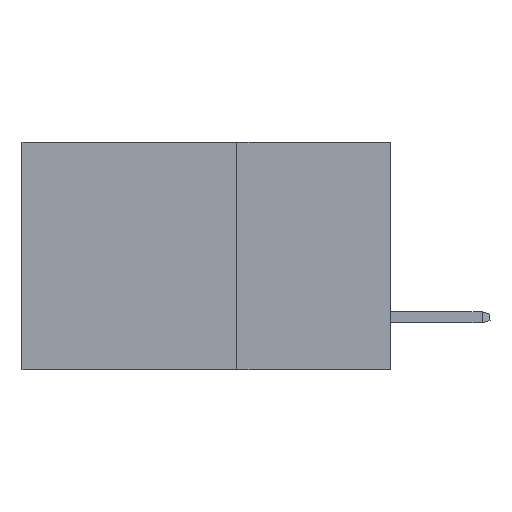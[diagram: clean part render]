
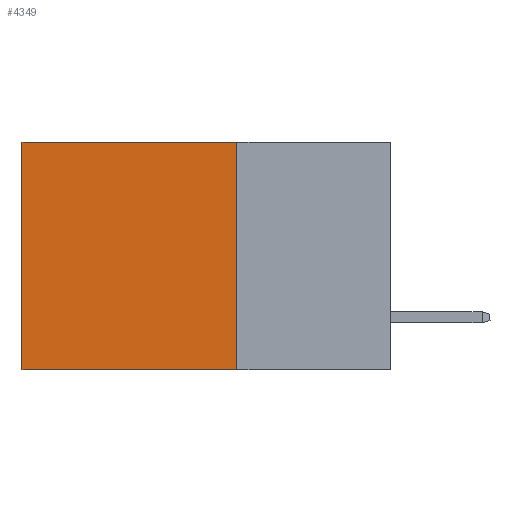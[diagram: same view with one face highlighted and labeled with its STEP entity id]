
A CAD part, left-side view. The second image highlights one B-rep face of the part: STEP entity #4349.
In plain terms, the highlighted planar face has unit normal (-1, 0, 0).
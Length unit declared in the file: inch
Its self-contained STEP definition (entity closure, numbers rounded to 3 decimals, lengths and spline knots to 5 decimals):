
#86 = VERTEX_POINT ( 'NONE', #23650 ) ;
#901 = PLANE ( 'NONE',  #24471 ) ;
#1737 = VECTOR ( 'NONE', #8459, 39.37008 ) ;
#2814 = EDGE_LOOP ( 'NONE', ( #7175, #16701, #22996, #6249 ) ) ;
#3805 = DIRECTION ( 'NONE',  ( 0., 0., -1. ) ) ;
#4349 = ADVANCED_FACE ( 'NONE', ( #18020 ), #901, .F. ) ;
#4884 = DIRECTION ( 'NONE',  ( 1., 0., 0. ) ) ;
#6249 = ORIENTED_EDGE ( 'NONE', *, *, #23647, .T. ) ;
#7019 = LINE ( 'NONE', #23610, #1737 ) ;
#7062 = VECTOR ( 'NONE', #3805, 39.37008 ) ;
#7175 = ORIENTED_EDGE ( 'NONE', *, *, #10825, .T. ) ;
#7646 = DIRECTION ( 'NONE',  ( 0., 1., 0. ) ) ;
#8459 = DIRECTION ( 'NONE',  ( 0., 1., 0. ) ) ;
#8644 = LINE ( 'NONE', #11830, #13734 ) ;
#9394 = VECTOR ( 'NONE', #7646, 39.37008 ) ;
#9986 = DIRECTION ( 'NONE',  ( 0., 0., -1. ) ) ;
#10220 = CARTESIAN_POINT ( 'NONE',  ( 0.2875, 0.25, -0.37 ) ) ;
#10825 = EDGE_CURVE ( 'NONE', #15213, #86, #8644, .T. ) ;
#11583 = CARTESIAN_POINT ( 'NONE',  ( 0.2875, 0.25, 0. ) ) ;
#11830 = CARTESIAN_POINT ( 'NONE',  ( 0.2875, 0.6, 0. ) ) ;
#12175 = LINE ( 'NONE', #11583, #7062 ) ;
#13734 = VECTOR ( 'NONE', #9986, 39.37008 ) ;
#14250 = EDGE_CURVE ( 'NONE', #20276, #86, #19507, .T. ) ;
#15213 = VERTEX_POINT ( 'NONE', #24334 ) ;
#15412 = VERTEX_POINT ( 'NONE', #17369 ) ;
#16066 = EDGE_CURVE ( 'NONE', #15412, #20276, #12175, .T. ) ;
#16452 = CARTESIAN_POINT ( 'NONE',  ( 0.2875, 0.25, 0. ) ) ;
#16701 = ORIENTED_EDGE ( 'NONE', *, *, #14250, .F. ) ;
#17369 = CARTESIAN_POINT ( 'NONE',  ( 0.2875, 0.25, 0. ) ) ;
#18020 = FACE_OUTER_BOUND ( 'NONE', #2814, .T. ) ;
#18334 = DIRECTION ( 'NONE',  ( 0., 0., -1. ) ) ;
#19507 = LINE ( 'NONE', #20987, #9394 ) ;
#20276 = VERTEX_POINT ( 'NONE', #10220 ) ;
#20987 = CARTESIAN_POINT ( 'NONE',  ( 0.2875, 0.25, -0.37 ) ) ;
#22996 = ORIENTED_EDGE ( 'NONE', *, *, #16066, .F. ) ;
#23610 = CARTESIAN_POINT ( 'NONE',  ( 0.2875, 0.25, 0. ) ) ;
#23647 = EDGE_CURVE ( 'NONE', #15412, #15213, #7019, .T. ) ;
#23650 = CARTESIAN_POINT ( 'NONE',  ( 0.2875, 0.6, -0.37 ) ) ;
#24334 = CARTESIAN_POINT ( 'NONE',  ( 0.2875, 0.6, 0. ) ) ;
#24471 = AXIS2_PLACEMENT_3D ( 'NONE', #16452, #4884, #18334 ) ;
